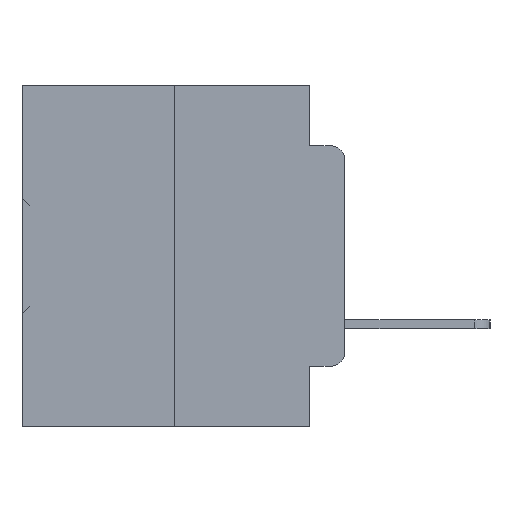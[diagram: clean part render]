
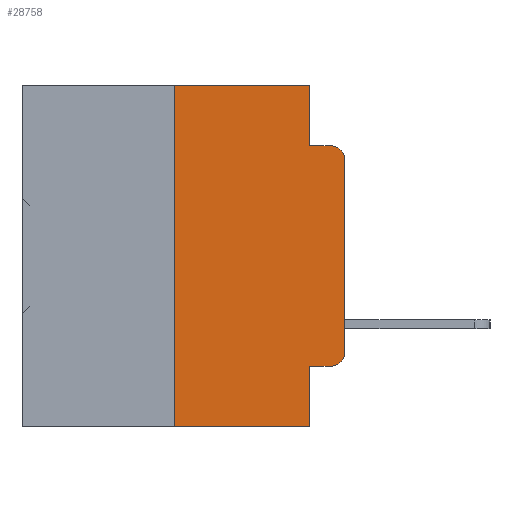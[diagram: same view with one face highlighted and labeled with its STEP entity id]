
A CAD part, left-side view. The second image highlights one B-rep face of the part: STEP entity #28758.
In plain terms, the highlighted planar face has unit normal (-1, 0, 0).
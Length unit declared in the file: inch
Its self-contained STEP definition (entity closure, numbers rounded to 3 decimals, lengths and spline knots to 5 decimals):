
#454 = CARTESIAN_POINT ( 'NONE',  ( 0., 0.02, -0.1085 ) ) ;
#636 = EDGE_CURVE ( 'NONE', #18967, #36869, #28047, .T. ) ;
#716 = EDGE_CURVE ( 'NONE', #19435, #24000, #32996, .T. ) ;
#759 = DIRECTION ( 'NONE',  ( 0., -1., 0. ) ) ;
#868 = CIRCLE ( 'NONE', #18763, 0.02 ) ;
#3220 = ORIENTED_EDGE ( 'NONE', *, *, #10551, .F. ) ;
#3410 = DIRECTION ( 'NONE',  ( 0., 0., -1. ) ) ;
#3882 = CARTESIAN_POINT ( 'NONE',  ( 0., 0.051, -0.0885 ) ) ;
#4149 = DIRECTION ( 'NONE',  ( 0., 0., 1. ) ) ;
#4568 = CARTESIAN_POINT ( 'NONE',  ( 0., 0.473, -0.5 ) ) ;
#4672 = CARTESIAN_POINT ( 'NONE',  ( 0., 0.051, -0.0885 ) ) ;
#5308 = VERTEX_POINT ( 'NONE', #3882 ) ;
#6067 = CARTESIAN_POINT ( 'NONE',  ( 0., 0.051, 0. ) ) ;
#6622 = CARTESIAN_POINT ( 'NONE',  ( 0., 0.051, -0.4115 ) ) ;
#7082 = CIRCLE ( 'NONE', #27091, 0.02 ) ;
#7105 = ORIENTED_EDGE ( 'NONE', *, *, #29274, .F. ) ;
#7502 = DIRECTION ( 'NONE',  ( 0., -1., 0. ) ) ;
#7567 = ORIENTED_EDGE ( 'NONE', *, *, #17624, .F. ) ;
#7610 = DIRECTION ( 'NONE',  ( 0., -1., 0. ) ) ;
#8054 = EDGE_CURVE ( 'NONE', #24000, #16192, #7082, .T. ) ;
#8611 = VERTEX_POINT ( 'NONE', #17283 ) ;
#8954 = ORIENTED_EDGE ( 'NONE', *, *, #15640, .F. ) ;
#9779 = VERTEX_POINT ( 'NONE', #28873 ) ;
#9867 = VECTOR ( 'NONE', #21216, 39.37008 ) ;
#10551 = EDGE_CURVE ( 'NONE', #36869, #5308, #26040, .T. ) ;
#11212 = ORIENTED_EDGE ( 'NONE', *, *, #716, .T. ) ;
#11878 = CARTESIAN_POINT ( 'NONE',  ( 0., 0.473, 0. ) ) ;
#12039 = CARTESIAN_POINT ( 'NONE',  ( 0., 0.051, 0. ) ) ;
#12816 = CARTESIAN_POINT ( 'NONE',  ( 0., 0., -0.3915 ) ) ;
#13459 = EDGE_LOOP ( 'NONE', ( #11212, #18847, #8954, #3220, #35124, #7567, #18076, #7105, #13543, #23138 ) ) ;
#13543 = ORIENTED_EDGE ( 'NONE', *, *, #31224, .T. ) ;
#13787 = LINE ( 'NONE', #6622, #20633 ) ;
#13929 = DIRECTION ( 'NONE',  ( -1., 0., 0. ) ) ;
#13959 = VERTEX_POINT ( 'NONE', #25408 ) ;
#14127 = AXIS2_PLACEMENT_3D ( 'NONE', #11878, #32181, #14796 ) ;
#14406 = LINE ( 'NONE', #25847, #29822 ) ;
#14796 = DIRECTION ( 'NONE',  ( 0., 0., -1. ) ) ;
#15075 = DIRECTION ( 'NONE',  ( 0., 0., -1. ) ) ;
#15640 = EDGE_CURVE ( 'NONE', #5308, #16192, #29434, .T. ) ;
#16022 = VERTEX_POINT ( 'NONE', #23766 ) ;
#16192 = VERTEX_POINT ( 'NONE', #18680 ) ;
#17283 = CARTESIAN_POINT ( 'NONE',  ( 0., 0.25, -0.5 ) ) ;
#17624 = EDGE_CURVE ( 'NONE', #8611, #18967, #35471, .T. ) ;
#18076 = ORIENTED_EDGE ( 'NONE', *, *, #29060, .T. ) ;
#18680 = CARTESIAN_POINT ( 'NONE',  ( 0., 0.02, -0.0885 ) ) ;
#18763 = AXIS2_PLACEMENT_3D ( 'NONE', #31317, #13929, #34183 ) ;
#18847 = ORIENTED_EDGE ( 'NONE', *, *, #8054, .T. ) ;
#18967 = VERTEX_POINT ( 'NONE', #25082 ) ;
#19435 = VERTEX_POINT ( 'NONE', #12816 ) ;
#20123 = DIRECTION ( 'NONE',  ( 0., 0., -1. ) ) ;
#20149 = VECTOR ( 'NONE', #4149, 39.37008 ) ;
#20633 = VECTOR ( 'NONE', #759, 39.37008 ) ;
#20878 = DIRECTION ( 'NONE',  ( -1., 0., 0. ) ) ;
#21216 = DIRECTION ( 'NONE',  ( 0., 0., 1. ) ) ;
#21250 = VECTOR ( 'NONE', #22049, 39.37008 ) ;
#21266 = CARTESIAN_POINT ( 'NONE',  ( 0., 0., 0. ) ) ;
#22049 = DIRECTION ( 'NONE',  ( 0., -1., 0. ) ) ;
#22096 = CARTESIAN_POINT ( 'NONE',  ( 0., 0.473, 0. ) ) ;
#23138 = ORIENTED_EDGE ( 'NONE', *, *, #28572, .T. ) ;
#23766 = CARTESIAN_POINT ( 'NONE',  ( 0., 0.02, -0.4115 ) ) ;
#24000 = VERTEX_POINT ( 'NONE', #36389 ) ;
#25082 = CARTESIAN_POINT ( 'NONE',  ( 0., 0.25, 0. ) ) ;
#25408 = CARTESIAN_POINT ( 'NONE',  ( 0., 0.051, -0.5 ) ) ;
#25847 = CARTESIAN_POINT ( 'NONE',  ( 0., 0.051, 0. ) ) ;
#26040 = LINE ( 'NONE', #12039, #32782 ) ;
#27091 = AXIS2_PLACEMENT_3D ( 'NONE', #454, #20878, #3410 ) ;
#27437 = CARTESIAN_POINT ( 'NONE',  ( 0., 0.25, 0. ) ) ;
#28047 = LINE ( 'NONE', #22096, #21250 ) ;
#28572 = EDGE_CURVE ( 'NONE', #16022, #19435, #868, .T. ) ;
#28758 = ADVANCED_FACE ( 'NONE', ( #32273 ), #34921, .F. ) ;
#28873 = CARTESIAN_POINT ( 'NONE',  ( 0., 0.051, -0.4115 ) ) ;
#29060 = EDGE_CURVE ( 'NONE', #8611, #13959, #36742, .T. ) ;
#29095 = VECTOR ( 'NONE', #7502, 39.37008 ) ;
#29274 = EDGE_CURVE ( 'NONE', #9779, #13959, #14406, .T. ) ;
#29434 = LINE ( 'NONE', #4672, #36168 ) ;
#29822 = VECTOR ( 'NONE', #20123, 39.37008 ) ;
#31224 = EDGE_CURVE ( 'NONE', #9779, #16022, #13787, .T. ) ;
#31317 = CARTESIAN_POINT ( 'NONE',  ( 0., 0.02, -0.3915 ) ) ;
#32181 = DIRECTION ( 'NONE',  ( 1., 0., 0. ) ) ;
#32273 = FACE_OUTER_BOUND ( 'NONE', #13459, .T. ) ;
#32782 = VECTOR ( 'NONE', #15075, 39.37008 ) ;
#32996 = LINE ( 'NONE', #21266, #9867 ) ;
#34183 = DIRECTION ( 'NONE',  ( 0., 0., -1. ) ) ;
#34921 = PLANE ( 'NONE',  #14127 ) ;
#35124 = ORIENTED_EDGE ( 'NONE', *, *, #636, .F. ) ;
#35471 = LINE ( 'NONE', #27437, #20149 ) ;
#36168 = VECTOR ( 'NONE', #7610, 39.37008 ) ;
#36389 = CARTESIAN_POINT ( 'NONE',  ( 0., 0., -0.1085 ) ) ;
#36742 = LINE ( 'NONE', #4568, #29095 ) ;
#36869 = VERTEX_POINT ( 'NONE', #6067 ) ;
